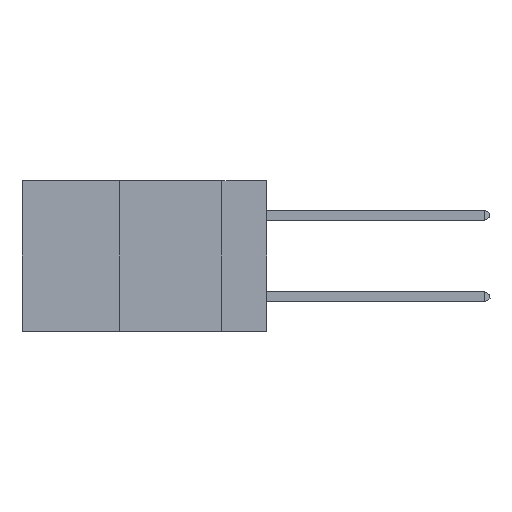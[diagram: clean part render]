
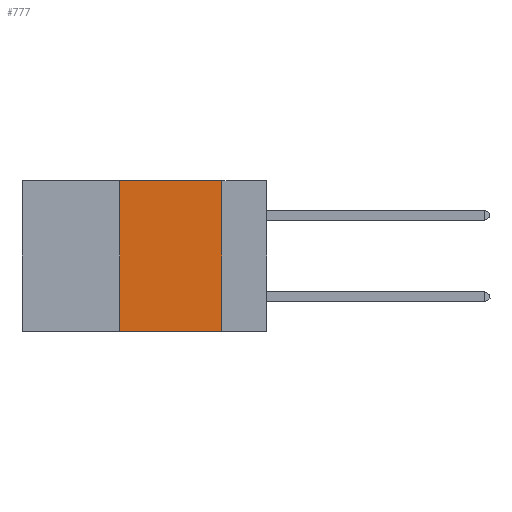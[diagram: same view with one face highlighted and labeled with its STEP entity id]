
A CAD part, left-side view. The second image highlights one B-rep face of the part: STEP entity #777.
In plain terms, the highlighted planar face has unit normal (-1, 0, 0).
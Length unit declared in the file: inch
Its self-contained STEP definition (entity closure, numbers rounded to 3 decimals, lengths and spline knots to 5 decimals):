
#422 = CARTESIAN_POINT ( 'NONE',  ( 0., 0.36, 0. ) ) ;
#504 = FACE_OUTER_BOUND ( 'NONE', #1689, .T. ) ;
#777 = ADVANCED_FACE ( 'NONE', ( #504 ), #3331, .F. ) ;
#801 = ORIENTED_EDGE ( 'NONE', *, *, #16181, .F. ) ;
#1080 = DIRECTION ( 'NONE',  ( 0., -1., 0. ) ) ;
#1181 = DIRECTION ( 'NONE',  ( 0., 0., -1. ) ) ;
#1232 = ORIENTED_EDGE ( 'NONE', *, *, #5823, .F. ) ;
#1689 = EDGE_LOOP ( 'NONE', ( #8611, #1232, #801, #14736 ) ) ;
#2672 = VECTOR ( 'NONE', #1181, 39.37008 ) ;
#2703 = VERTEX_POINT ( 'NONE', #10259 ) ;
#3218 = DIRECTION ( 'NONE',  ( 0., 0., -1. ) ) ;
#3331 = PLANE ( 'NONE',  #5535 ) ;
#3648 = VERTEX_POINT ( 'NONE', #7809 ) ;
#3835 = DIRECTION ( 'NONE',  ( 0., 0., 1. ) ) ;
#4815 = EDGE_CURVE ( 'NONE', #14204, #2703, #10336, .T. ) ;
#5120 = CARTESIAN_POINT ( 'NONE',  ( 0., 0.36, 0. ) ) ;
#5535 = AXIS2_PLACEMENT_3D ( 'NONE', #10347, #8464, #3218 ) ;
#5823 = EDGE_CURVE ( 'NONE', #11008, #3648, #7475, .T. ) ;
#6246 = LINE ( 'NONE', #5120, #12692 ) ;
#7051 = CARTESIAN_POINT ( 'NONE',  ( 0., 0.6, 0. ) ) ;
#7064 = VECTOR ( 'NONE', #12434, 39.37008 ) ;
#7475 = LINE ( 'NONE', #7051, #7064 ) ;
#7809 = CARTESIAN_POINT ( 'NONE',  ( 0., 0.11, 0. ) ) ;
#8464 = DIRECTION ( 'NONE',  ( 1., 0., 0. ) ) ;
#8611 = ORIENTED_EDGE ( 'NONE', *, *, #10726, .F. ) ;
#8917 = CARTESIAN_POINT ( 'NONE',  ( 0., 0.6, -0.37 ) ) ;
#10259 = CARTESIAN_POINT ( 'NONE',  ( 0., 0.11, -0.37 ) ) ;
#10279 = CARTESIAN_POINT ( 'NONE',  ( 0., 0.11, 0. ) ) ;
#10336 = LINE ( 'NONE', #8917, #16863 ) ;
#10347 = CARTESIAN_POINT ( 'NONE',  ( 0., 0.6, 0. ) ) ;
#10726 = EDGE_CURVE ( 'NONE', #3648, #2703, #15644, .T. ) ;
#11008 = VERTEX_POINT ( 'NONE', #422 ) ;
#12434 = DIRECTION ( 'NONE',  ( 0., -1., 0. ) ) ;
#12692 = VECTOR ( 'NONE', #3835, 39.37008 ) ;
#13341 = CARTESIAN_POINT ( 'NONE',  ( 0., 0.36, -0.37 ) ) ;
#14204 = VERTEX_POINT ( 'NONE', #13341 ) ;
#14736 = ORIENTED_EDGE ( 'NONE', *, *, #4815, .T. ) ;
#15644 = LINE ( 'NONE', #10279, #2672 ) ;
#16181 = EDGE_CURVE ( 'NONE', #14204, #11008, #6246, .T. ) ;
#16863 = VECTOR ( 'NONE', #1080, 39.37008 ) ;
